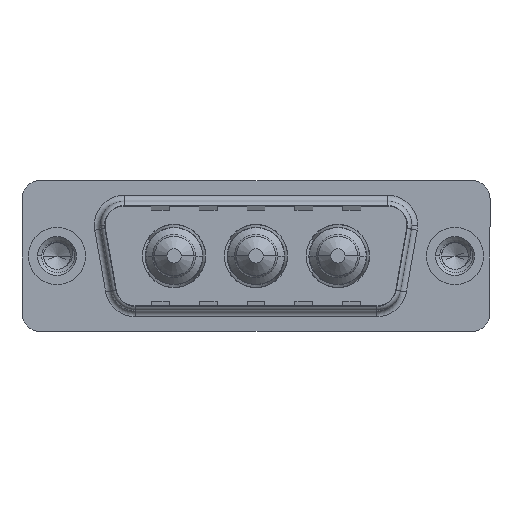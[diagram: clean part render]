
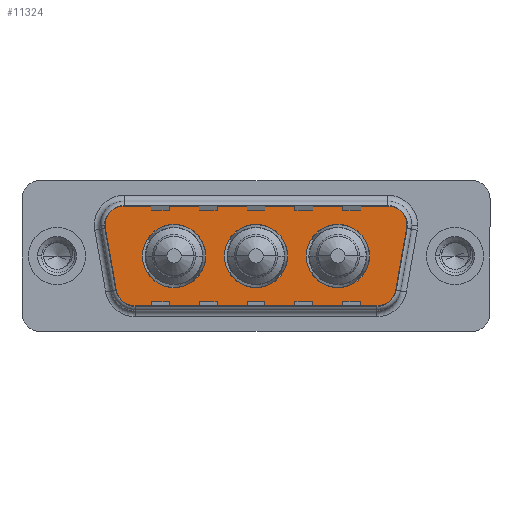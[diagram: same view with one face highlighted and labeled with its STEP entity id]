
A CAD part, top view. The second image highlights one B-rep face of the part: STEP entity #11324.
In plain terms, the highlighted planar face has unit normal (0, 0, 1).
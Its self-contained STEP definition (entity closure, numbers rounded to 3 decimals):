
#48 = CIRCLE ( 'NONE', #12399, 2.65 ) ;
#158 = EDGE_CURVE ( 'NONE', #5331, #4299, #11968, .T. ) ;
#306 = LINE ( 'NONE', #10063, #5600 ) ;
#326 = PLANE ( 'NONE',  #2355 ) ;
#524 = VERTEX_POINT ( 'NONE', #13225 ) ;
#641 = DIRECTION ( 'NONE',  ( 0., 0., 1. ) ) ;
#761 = FACE_BOUND ( 'NONE', #1579, .T. ) ;
#798 = CIRCLE ( 'NONE', #7593, 2. ) ;
#1067 = EDGE_LOOP ( 'NONE', ( #9182, #9407 ) ) ;
#1238 = ORIENTED_EDGE ( 'NONE', *, *, #3816, .T. ) ;
#1330 = EDGE_CURVE ( 'NONE', #1774, #13740, #9160, .T. ) ;
#1552 = DIRECTION ( 'NONE',  ( 0., 0., 1. ) ) ;
#1563 = CIRCLE ( 'NONE', #8360, 2. ) ;
#1573 = CARTESIAN_POINT ( 'NONE',  ( 26.866, -2.9, 0. ) ) ;
#1579 = EDGE_LOOP ( 'NONE', ( #2257, #9531 ) ) ;
#1680 = AXIS2_PLACEMENT_3D ( 'NONE', #6207, #2009, #13273 ) ;
#1774 = VERTEX_POINT ( 'NONE', #4340 ) ;
#1844 = CARTESIAN_POINT ( 'NONE',  ( 28.836, -3.247, 0. ) ) ;
#2009 = DIRECTION ( 'NONE',  ( 0., 0., 1. ) ) ;
#2044 = EDGE_CURVE ( 'NONE', #7402, #13510, #11581, .T. ) ;
#2162 = DIRECTION ( 'NONE',  ( 1., 0., 0. ) ) ;
#2164 = CIRCLE ( 'NONE', #9165, 2.65 ) ;
#2257 = ORIENTED_EDGE ( 'NONE', *, *, #1330, .F. ) ;
#2355 = AXIS2_PLACEMENT_3D ( 'NONE', #2543, #12053, #5695 ) ;
#2398 = ORIENTED_EDGE ( 'NONE', *, *, #8651, .T. ) ;
#2416 = ORIENTED_EDGE ( 'NONE', *, *, #4079, .F. ) ;
#2453 = DIRECTION ( 'NONE',  ( 1., 0., 0. ) ) ;
#2523 = EDGE_CURVE ( 'NONE', #11769, #5648, #306, .T. ) ;
#2543 = CARTESIAN_POINT ( 'NONE',  ( 26.866, -2.9, 0. ) ) ;
#2575 = CARTESIAN_POINT ( 'NONE',  ( 6.434, -2.9, 0. ) ) ;
#2625 = AXIS2_PLACEMENT_3D ( 'NONE', #13672, #11437, #11668 ) ;
#2766 = CARTESIAN_POINT ( 'NONE',  ( 27.889, 2.9, 0. ) ) ;
#2890 = CARTESIAN_POINT ( 'NONE',  ( 27.889, 4.9, 0. ) ) ;
#2923 = CARTESIAN_POINT ( 'NONE',  ( 20.85, 0., 0. ) ) ;
#3236 = CARTESIAN_POINT ( 'NONE',  ( 23.5, 0., 0. ) ) ;
#3241 = CARTESIAN_POINT ( 'NONE',  ( 6.434, -4.9, 0. ) ) ;
#3245 = FACE_BOUND ( 'NONE', #1067, .T. ) ;
#3356 = VECTOR ( 'NONE', #6593, 1000. ) ;
#3382 = CIRCLE ( 'NONE', #10663, 2.65 ) ;
#3425 = DIRECTION ( 'NONE',  ( 0.174, -0.985, 0. ) ) ;
#3497 = VERTEX_POINT ( 'NONE', #13608 ) ;
#3638 = ORIENTED_EDGE ( 'NONE', *, *, #12473, .T. ) ;
#3666 = CARTESIAN_POINT ( 'NONE',  ( 9.8, 0., 0. ) ) ;
#3722 = CIRCLE ( 'NONE', #4743, 2. ) ;
#3793 = CARTESIAN_POINT ( 'NONE',  ( 4.464, -3.247, 0. ) ) ;
#3810 = DIRECTION ( 'NONE',  ( -1., 0., 0. ) ) ;
#3816 = EDGE_CURVE ( 'NONE', #5648, #8829, #798, .T. ) ;
#3918 = EDGE_CURVE ( 'NONE', #5849, #3497, #10683, .T. ) ;
#3940 = DIRECTION ( 'NONE',  ( 0., 0., 1. ) ) ;
#3972 = CARTESIAN_POINT ( 'NONE',  ( 5.411, 4.9, 0. ) ) ;
#4079 = EDGE_CURVE ( 'NONE', #6543, #7264, #6550, .T. ) ;
#4299 = VERTEX_POINT ( 'NONE', #10552 ) ;
#4340 = CARTESIAN_POINT ( 'NONE',  ( 19.3, 0., 0. ) ) ;
#4344 = CARTESIAN_POINT ( 'NONE',  ( 27.889, 2.9, 0. ) ) ;
#4743 = AXIS2_PLACEMENT_3D ( 'NONE', #2766, #10143, #3810 ) ;
#5002 = VECTOR ( 'NONE', #7898, 1000. ) ;
#5331 = VERTEX_POINT ( 'NONE', #11826 ) ;
#5434 = EDGE_LOOP ( 'NONE', ( #7081, #3638, #8911, #12278, #2398, #7602, #12955, #1238, #9169 ) ) ;
#5515 = EDGE_CURVE ( 'NONE', #7264, #6543, #48, .T. ) ;
#5600 = VECTOR ( 'NONE', #3425, 1000. ) ;
#5648 = VERTEX_POINT ( 'NONE', #3793 ) ;
#5695 = DIRECTION ( 'NONE',  ( 1., 0., 0. ) ) ;
#5725 = CARTESIAN_POINT ( 'NONE',  ( 7.15, 0., 0. ) ) ;
#5747 = EDGE_CURVE ( 'NONE', #3497, #5849, #3382, .T. ) ;
#5849 = VERTEX_POINT ( 'NONE', #2923 ) ;
#6149 = LINE ( 'NONE', #11019, #3356 ) ;
#6207 = CARTESIAN_POINT ( 'NONE',  ( 23.5, 0., 0. ) ) ;
#6289 = CARTESIAN_POINT ( 'NONE',  ( 29.859, 2.553, 0. ) ) ;
#6306 = CARTESIAN_POINT ( 'NONE',  ( 3.441, 2.553, 0. ) ) ;
#6316 = VERTEX_POINT ( 'NONE', #2890 ) ;
#6357 = FACE_OUTER_BOUND ( 'NONE', #5434, .T. ) ;
#6506 = DIRECTION ( 'NONE',  ( -1., 0., 0. ) ) ;
#6531 = DIRECTION ( 'NONE',  ( 0., 0., 1. ) ) ;
#6543 = VERTEX_POINT ( 'NONE', #9269 ) ;
#6550 = CIRCLE ( 'NONE', #10149, 2.65 ) ;
#6593 = DIRECTION ( 'NONE',  ( 1., 0., 0. ) ) ;
#6779 = EDGE_CURVE ( 'NONE', #8829, #7402, #6149, .T. ) ;
#6947 = CARTESIAN_POINT ( 'NONE',  ( 16.65, 0., 0. ) ) ;
#7081 = ORIENTED_EDGE ( 'NONE', *, *, #2044, .T. ) ;
#7151 = DIRECTION ( 'NONE',  ( 1., 0., 0. ) ) ;
#7215 = DIRECTION ( 'NONE',  ( 0., 0., 1. ) ) ;
#7264 = VERTEX_POINT ( 'NONE', #5725 ) ;
#7402 = VERTEX_POINT ( 'NONE', #12902 ) ;
#7593 = AXIS2_PLACEMENT_3D ( 'NONE', #2575, #13477, #12412 ) ;
#7602 = ORIENTED_EDGE ( 'NONE', *, *, #8197, .T. ) ;
#7664 = DIRECTION ( 'NONE',  ( 0., 0., 1. ) ) ;
#7864 = LINE ( 'NONE', #3972, #5002 ) ;
#7898 = DIRECTION ( 'NONE',  ( -1., 0., 0. ) ) ;
#8091 = DIRECTION ( 'NONE',  ( 1., 0., 0. ) ) ;
#8197 = EDGE_CURVE ( 'NONE', #524, #11769, #1563, .T. ) ;
#8282 = CARTESIAN_POINT ( 'NONE',  ( 9.8, 0., 0. ) ) ;
#8360 = AXIS2_PLACEMENT_3D ( 'NONE', #11832, #7215, #7151 ) ;
#8651 = EDGE_CURVE ( 'NONE', #6316, #524, #7864, .T. ) ;
#8829 = VERTEX_POINT ( 'NONE', #3241 ) ;
#8907 = FACE_BOUND ( 'NONE', #9391, .T. ) ;
#8911 = ORIENTED_EDGE ( 'NONE', *, *, #158, .T. ) ;
#9125 = DIRECTION ( 'NONE',  ( 1., 0., 0. ) ) ;
#9160 = CIRCLE ( 'NONE', #2625, 2.65 ) ;
#9165 = AXIS2_PLACEMENT_3D ( 'NONE', #6947, #641, #8091 ) ;
#9169 = ORIENTED_EDGE ( 'NONE', *, *, #6779, .T. ) ;
#9182 = ORIENTED_EDGE ( 'NONE', *, *, #5747, .F. ) ;
#9269 = CARTESIAN_POINT ( 'NONE',  ( 12.45, 0., 0. ) ) ;
#9391 = EDGE_LOOP ( 'NONE', ( #2416, #13335 ) ) ;
#9407 = ORIENTED_EDGE ( 'NONE', *, *, #3918, .F. ) ;
#9503 = EDGE_CURVE ( 'NONE', #13740, #1774, #2164, .T. ) ;
#9531 = ORIENTED_EDGE ( 'NONE', *, *, #9503, .F. ) ;
#10063 = CARTESIAN_POINT ( 'NONE',  ( 3.441, 2.553, 0. ) ) ;
#10143 = DIRECTION ( 'NONE',  ( 0., 0., 1. ) ) ;
#10149 = AXIS2_PLACEMENT_3D ( 'NONE', #3666, #10224, #13398 ) ;
#10224 = DIRECTION ( 'NONE',  ( 0., 0., 1. ) ) ;
#10497 = VECTOR ( 'NONE', #13739, 1000. ) ;
#10552 = CARTESIAN_POINT ( 'NONE',  ( 29.889, 2.9, 0. ) ) ;
#10663 = AXIS2_PLACEMENT_3D ( 'NONE', #3236, #1552, #2162 ) ;
#10683 = CIRCLE ( 'NONE', #1680, 2.65 ) ;
#11019 = CARTESIAN_POINT ( 'NONE',  ( 6.434, -4.9, 0. ) ) ;
#11177 = CARTESIAN_POINT ( 'NONE',  ( 14., 0., 0. ) ) ;
#11267 = AXIS2_PLACEMENT_3D ( 'NONE', #1573, #3940, #2453 ) ;
#11324 = ADVANCED_FACE ( 'NONE', ( #761, #3245, #8907, #6357 ), #326, .T. ) ;
#11437 = DIRECTION ( 'NONE',  ( 0., 0., 1. ) ) ;
#11581 = CIRCLE ( 'NONE', #11267, 2. ) ;
#11668 = DIRECTION ( 'NONE',  ( 1., 0., 0. ) ) ;
#11702 = AXIS2_PLACEMENT_3D ( 'NONE', #4344, #6531, #6506 ) ;
#11769 = VERTEX_POINT ( 'NONE', #6306 ) ;
#11826 = CARTESIAN_POINT ( 'NONE',  ( 29.859, 2.553, 0. ) ) ;
#11832 = CARTESIAN_POINT ( 'NONE',  ( 5.411, 2.9, 0. ) ) ;
#11834 = LINE ( 'NONE', #6289, #10497 ) ;
#11968 = CIRCLE ( 'NONE', #11702, 2. ) ;
#12053 = DIRECTION ( 'NONE',  ( 0., 0., 1. ) ) ;
#12278 = ORIENTED_EDGE ( 'NONE', *, *, #12927, .T. ) ;
#12399 = AXIS2_PLACEMENT_3D ( 'NONE', #8282, #7664, #9125 ) ;
#12412 = DIRECTION ( 'NONE',  ( -1., 0., 0. ) ) ;
#12473 = EDGE_CURVE ( 'NONE', #13510, #5331, #11834, .T. ) ;
#12902 = CARTESIAN_POINT ( 'NONE',  ( 26.866, -4.9, 0. ) ) ;
#12927 = EDGE_CURVE ( 'NONE', #4299, #6316, #3722, .T. ) ;
#12955 = ORIENTED_EDGE ( 'NONE', *, *, #2523, .T. ) ;
#13225 = CARTESIAN_POINT ( 'NONE',  ( 5.411, 4.9, 0. ) ) ;
#13273 = DIRECTION ( 'NONE',  ( 1., 0., 0. ) ) ;
#13335 = ORIENTED_EDGE ( 'NONE', *, *, #5515, .F. ) ;
#13398 = DIRECTION ( 'NONE',  ( 1., 0., 0. ) ) ;
#13477 = DIRECTION ( 'NONE',  ( 0., 0., 1. ) ) ;
#13510 = VERTEX_POINT ( 'NONE', #1844 ) ;
#13608 = CARTESIAN_POINT ( 'NONE',  ( 26.15, 0., 0. ) ) ;
#13672 = CARTESIAN_POINT ( 'NONE',  ( 16.65, 0., 0. ) ) ;
#13739 = DIRECTION ( 'NONE',  ( 0.174, 0.985, 0. ) ) ;
#13740 = VERTEX_POINT ( 'NONE', #11177 ) ;
